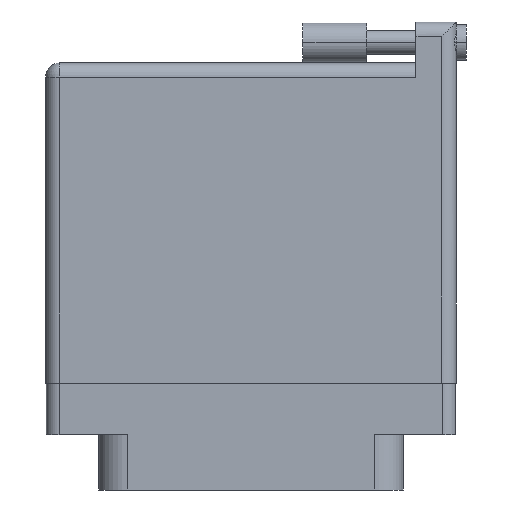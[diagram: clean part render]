
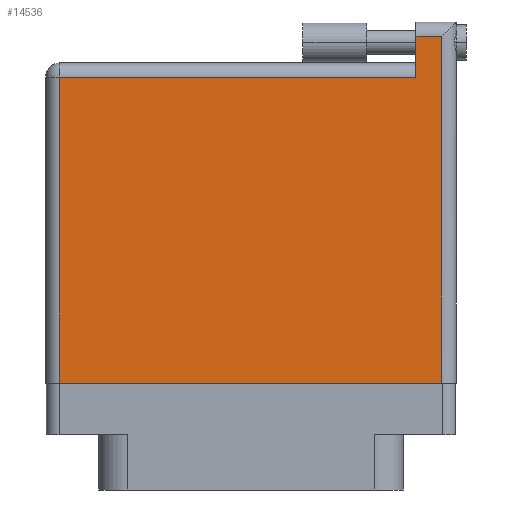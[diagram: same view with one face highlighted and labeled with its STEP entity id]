
A CAD part, front view. The second image highlights one B-rep face of the part: STEP entity #14536.
In plain terms, the highlighted face is planar.
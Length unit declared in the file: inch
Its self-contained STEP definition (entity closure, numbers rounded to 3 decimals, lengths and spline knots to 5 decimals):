
#2373 = VECTOR ( 'NONE', #24397, 39.37008 ) ;
#2447 = DIRECTION ( 'NONE',  ( -1., 0., 0. ) ) ;
#3532 = LINE ( 'NONE', #29452, #33397 ) ;
#4196 = CARTESIAN_POINT ( 'NONE',  ( -1.004, -0.1, 0.4495 ) ) ;
#4326 = FACE_OUTER_BOUND ( 'NONE', #27877, .T. ) ;
#4929 = LINE ( 'NONE', #21335, #19918 ) ;
#5200 = VERTEX_POINT ( 'NONE', #20917 ) ;
#5424 = CARTESIAN_POINT ( 'NONE',  ( -0.934, 1.396, 0.4495 ) ) ;
#8624 = CARTESIAN_POINT ( 'NONE',  ( 0.807, 1.596, 0.4495 ) ) ;
#11410 = DIRECTION ( 'NONE',  ( 0., 1., 0. ) ) ;
#11802 = ORIENTED_EDGE ( 'NONE', *, *, #36047, .T. ) ;
#12674 = EDGE_CURVE ( 'NONE', #27228, #5200, #25157, .T. ) ;
#13765 = LINE ( 'NONE', #23163, #20972 ) ;
#13867 = ORIENTED_EDGE ( 'NONE', *, *, #12674, .T. ) ;
#14536 = ADVANCED_FACE ( 'NONE', ( #4326 ), #14680, .F. ) ;
#14680 = PLANE ( 'NONE',  #20125 ) ;
#15509 = VERTEX_POINT ( 'NONE', #8624 ) ;
#16618 = VERTEX_POINT ( 'NONE', #30695 ) ;
#16820 = EDGE_CURVE ( 'NONE', #28430, #16618, #13765, .T. ) ;
#18336 = CARTESIAN_POINT ( 'NONE',  ( -1.004, 1.596, 0.4495 ) ) ;
#18380 = VECTOR ( 'NONE', #38108, 39.37008 ) ;
#18410 = EDGE_CURVE ( 'NONE', #15509, #38302, #3532, .T. ) ;
#18966 = CARTESIAN_POINT ( 'NONE',  ( -1.004, 1.466, 0.4495 ) ) ;
#19918 = VECTOR ( 'NONE', #2447, 39.37008 ) ;
#20125 = AXIS2_PLACEMENT_3D ( 'NONE', #18966, #34032, #25141 ) ;
#20270 = LINE ( 'NONE', #18336, #2373 ) ;
#20686 = CARTESIAN_POINT ( 'NONE',  ( 0.934, -0.1, 0.4495 ) ) ;
#20917 = CARTESIAN_POINT ( 'NONE',  ( 0.934, 1.596, 0.4495 ) ) ;
#20972 = VECTOR ( 'NONE', #26105, 39.37008 ) ;
#21186 = ORIENTED_EDGE ( 'NONE', *, *, #16820, .T. ) ;
#21335 = CARTESIAN_POINT ( 'NONE',  ( -1.004, 1.396, 0.4495 ) ) ;
#22136 = ORIENTED_EDGE ( 'NONE', *, *, #18410, .T. ) ;
#23163 = CARTESIAN_POINT ( 'NONE',  ( -0.934, -0.1, 0.4495 ) ) ;
#24397 = DIRECTION ( 'NONE',  ( -1., 0., 0. ) ) ;
#24977 = EDGE_CURVE ( 'NONE', #5200, #15509, #20270, .T. ) ;
#25141 = DIRECTION ( 'NONE',  ( -1., 0., 0. ) ) ;
#25157 = LINE ( 'NONE', #29852, #39573 ) ;
#26105 = DIRECTION ( 'NONE',  ( 0., -1., 0. ) ) ;
#27228 = VERTEX_POINT ( 'NONE', #20686 ) ;
#27877 = EDGE_LOOP ( 'NONE', ( #29421, #13867, #28270, #22136, #11802, #21186 ) ) ;
#28270 = ORIENTED_EDGE ( 'NONE', *, *, #24977, .T. ) ;
#28430 = VERTEX_POINT ( 'NONE', #5424 ) ;
#29421 = ORIENTED_EDGE ( 'NONE', *, *, #31819, .T. ) ;
#29452 = CARTESIAN_POINT ( 'NONE',  ( 0.807, 1.666, 0.4495 ) ) ;
#29852 = CARTESIAN_POINT ( 'NONE',  ( 0.934, 1.666, 0.4495 ) ) ;
#30695 = CARTESIAN_POINT ( 'NONE',  ( -0.934, -0.1, 0.4495 ) ) ;
#31819 = EDGE_CURVE ( 'NONE', #16618, #27228, #37141, .T. ) ;
#33397 = VECTOR ( 'NONE', #39608, 39.37008 ) ;
#34032 = DIRECTION ( 'NONE',  ( 0., 0., -1. ) ) ;
#35827 = CARTESIAN_POINT ( 'NONE',  ( 0.807, 1.396, 0.4495 ) ) ;
#36047 = EDGE_CURVE ( 'NONE', #38302, #28430, #4929, .T. ) ;
#37141 = LINE ( 'NONE', #4196, #18380 ) ;
#38108 = DIRECTION ( 'NONE',  ( 1., 0., 0. ) ) ;
#38302 = VERTEX_POINT ( 'NONE', #35827 ) ;
#39573 = VECTOR ( 'NONE', #11410, 39.37008 ) ;
#39608 = DIRECTION ( 'NONE',  ( 0., -1., 0. ) ) ;
